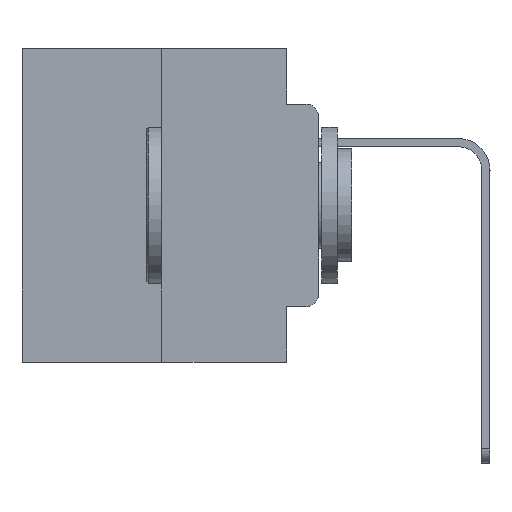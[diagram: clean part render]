
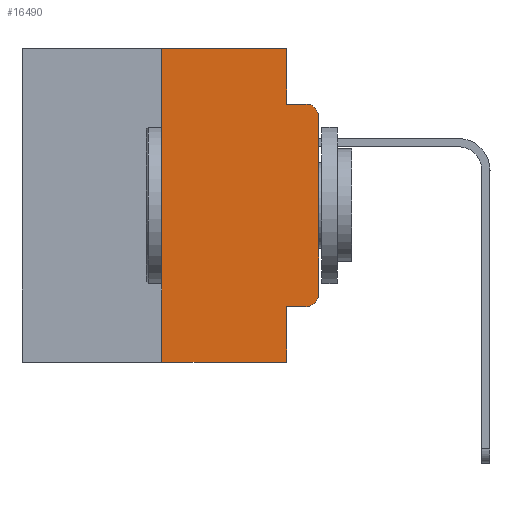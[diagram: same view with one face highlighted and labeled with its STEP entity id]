
A CAD part, left-side view. The second image highlights one B-rep face of the part: STEP entity #16490.
In plain terms, the highlighted planar face has unit normal (-1, 0, 0).
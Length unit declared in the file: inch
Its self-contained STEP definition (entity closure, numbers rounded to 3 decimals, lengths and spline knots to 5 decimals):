
#47 = EDGE_CURVE ( 'NONE', #20950, #2718, #7813, .T. ) ;
#105 = ORIENTED_EDGE ( 'NONE', *, *, #15860, .T. ) ;
#117 = EDGE_CURVE ( 'NONE', #18870, #1925, #6535, .T. ) ;
#793 = DIRECTION ( 'NONE',  ( 0., 0., -1. ) ) ;
#898 = CARTESIAN_POINT ( 'NONE',  ( 0., 0.02, -0.3915 ) ) ;
#969 = DIRECTION ( 'NONE',  ( 0., 0., 1. ) ) ;
#1144 = CARTESIAN_POINT ( 'NONE',  ( 0., 0., 0. ) ) ;
#1352 = EDGE_CURVE ( 'NONE', #2718, #24528, #23585, .T. ) ;
#1913 = ORIENTED_EDGE ( 'NONE', *, *, #3688, .T. ) ;
#1925 = VERTEX_POINT ( 'NONE', #26360 ) ;
#1959 = ORIENTED_EDGE ( 'NONE', *, *, #17411, .F. ) ;
#2378 = VECTOR ( 'NONE', #26526, 39.37008 ) ;
#2646 = VECTOR ( 'NONE', #25416, 39.37008 ) ;
#2718 = VERTEX_POINT ( 'NONE', #6064 ) ;
#3160 = CIRCLE ( 'NONE', #12914, 0.02 ) ;
#3595 = VECTOR ( 'NONE', #14387, 39.37008 ) ;
#3671 = LINE ( 'NONE', #9697, #2378 ) ;
#3688 = EDGE_CURVE ( 'NONE', #19106, #20929, #3671, .T. ) ;
#4253 = DIRECTION ( 'NONE',  ( 0., 0., -1. ) ) ;
#4764 = EDGE_CURVE ( 'NONE', #26649, #20950, #15291, .T. ) ;
#4878 = DIRECTION ( 'NONE',  ( 0., 0., -1. ) ) ;
#5120 = VECTOR ( 'NONE', #11595, 39.37008 ) ;
#5212 = EDGE_CURVE ( 'NONE', #25440, #26649, #9109, .T. ) ;
#5656 = CARTESIAN_POINT ( 'NONE',  ( 0., 0.051, -0.0885 ) ) ;
#5669 = VECTOR ( 'NONE', #4253, 39.37008 ) ;
#6064 = CARTESIAN_POINT ( 'NONE',  ( 0., 0.051, -0.0885 ) ) ;
#6531 = CARTESIAN_POINT ( 'NONE',  ( 0., 0.051, -0.4115 ) ) ;
#6535 = LINE ( 'NONE', #1144, #13011 ) ;
#6628 = EDGE_CURVE ( 'NONE', #20929, #18870, #3160, .T. ) ;
#6812 = CARTESIAN_POINT ( 'NONE',  ( 0., 0.473, 0. ) ) ;
#6995 = ORIENTED_EDGE ( 'NONE', *, *, #47, .F. ) ;
#7237 = PLANE ( 'NONE',  #13264 ) ;
#7813 = LINE ( 'NONE', #19124, #9754 ) ;
#8476 = CARTESIAN_POINT ( 'NONE',  ( 0., 0.051, 0. ) ) ;
#9109 = LINE ( 'NONE', #26771, #3595 ) ;
#9680 = ORIENTED_EDGE ( 'NONE', *, *, #1352, .F. ) ;
#9697 = CARTESIAN_POINT ( 'NONE',  ( 0., 0.051, -0.4115 ) ) ;
#9754 = VECTOR ( 'NONE', #13045, 39.37008 ) ;
#10107 = ORIENTED_EDGE ( 'NONE', *, *, #5212, .F. ) ;
#10197 = EDGE_LOOP ( 'NONE', ( #11864, #11975, #9680, #6995, #23642, #10107, #105, #1959, #1913, #26457 ) ) ;
#10331 = CARTESIAN_POINT ( 'NONE',  ( 0., 0.051, 0. ) ) ;
#10627 = LINE ( 'NONE', #26415, #5120 ) ;
#11027 = CARTESIAN_POINT ( 'NONE',  ( 0., 0.02, -0.1085 ) ) ;
#11595 = DIRECTION ( 'NONE',  ( 0., -1., 0. ) ) ;
#11864 = ORIENTED_EDGE ( 'NONE', *, *, #117, .T. ) ;
#11975 = ORIENTED_EDGE ( 'NONE', *, *, #14158, .T. ) ;
#12914 = AXIS2_PLACEMENT_3D ( 'NONE', #898, #17501, #4878 ) ;
#13011 = VECTOR ( 'NONE', #969, 39.37008 ) ;
#13045 = DIRECTION ( 'NONE',  ( 0., 0., -1. ) ) ;
#13264 = AXIS2_PLACEMENT_3D ( 'NONE', #23753, #21737, #15649 ) ;
#14158 = EDGE_CURVE ( 'NONE', #1925, #24528, #19519, .T. ) ;
#14387 = DIRECTION ( 'NONE',  ( 0., 0., 1. ) ) ;
#15291 = LINE ( 'NONE', #6812, #2646 ) ;
#15649 = DIRECTION ( 'NONE',  ( 0., 0., -1. ) ) ;
#15860 = EDGE_CURVE ( 'NONE', #25440, #20840, #10627, .T. ) ;
#16490 = ADVANCED_FACE ( 'NONE', ( #25242 ), #7237, .F. ) ;
#16524 = AXIS2_PLACEMENT_3D ( 'NONE', #11027, #19295, #793 ) ;
#17411 = EDGE_CURVE ( 'NONE', #19106, #20840, #21576, .T. ) ;
#17501 = DIRECTION ( 'NONE',  ( -1., 0., 0. ) ) ;
#18051 = CARTESIAN_POINT ( 'NONE',  ( 0., 0., -0.3915 ) ) ;
#18870 = VERTEX_POINT ( 'NONE', #18051 ) ;
#19106 = VERTEX_POINT ( 'NONE', #6531 ) ;
#19124 = CARTESIAN_POINT ( 'NONE',  ( 0., 0.051, 0. ) ) ;
#19295 = DIRECTION ( 'NONE',  ( -1., 0., 0. ) ) ;
#19519 = CIRCLE ( 'NONE', #16524, 0.02 ) ;
#19995 = DIRECTION ( 'NONE',  ( 0., -1., 0. ) ) ;
#20398 = CARTESIAN_POINT ( 'NONE',  ( 0., 0.051, -0.5 ) ) ;
#20840 = VERTEX_POINT ( 'NONE', #20398 ) ;
#20929 = VERTEX_POINT ( 'NONE', #25027 ) ;
#20950 = VERTEX_POINT ( 'NONE', #8476 ) ;
#21297 = VECTOR ( 'NONE', #19995, 39.37008 ) ;
#21576 = LINE ( 'NONE', #10331, #5669 ) ;
#21737 = DIRECTION ( 'NONE',  ( 1., 0., 0. ) ) ;
#22007 = CARTESIAN_POINT ( 'NONE',  ( 0., 0.02, -0.0885 ) ) ;
#23324 = CARTESIAN_POINT ( 'NONE',  ( 0., 0.25, 0. ) ) ;
#23477 = CARTESIAN_POINT ( 'NONE',  ( 0., 0.25, -0.5 ) ) ;
#23585 = LINE ( 'NONE', #5656, #21297 ) ;
#23642 = ORIENTED_EDGE ( 'NONE', *, *, #4764, .F. ) ;
#23753 = CARTESIAN_POINT ( 'NONE',  ( 0., 0.473, 0. ) ) ;
#24528 = VERTEX_POINT ( 'NONE', #22007 ) ;
#25027 = CARTESIAN_POINT ( 'NONE',  ( 0., 0.02, -0.4115 ) ) ;
#25242 = FACE_OUTER_BOUND ( 'NONE', #10197, .T. ) ;
#25416 = DIRECTION ( 'NONE',  ( 0., -1., 0. ) ) ;
#25440 = VERTEX_POINT ( 'NONE', #23477 ) ;
#26360 = CARTESIAN_POINT ( 'NONE',  ( 0., 0., -0.1085 ) ) ;
#26415 = CARTESIAN_POINT ( 'NONE',  ( 0., 0.473, -0.5 ) ) ;
#26457 = ORIENTED_EDGE ( 'NONE', *, *, #6628, .T. ) ;
#26526 = DIRECTION ( 'NONE',  ( 0., -1., 0. ) ) ;
#26649 = VERTEX_POINT ( 'NONE', #23324 ) ;
#26771 = CARTESIAN_POINT ( 'NONE',  ( 0., 0.25, 0. ) ) ;
